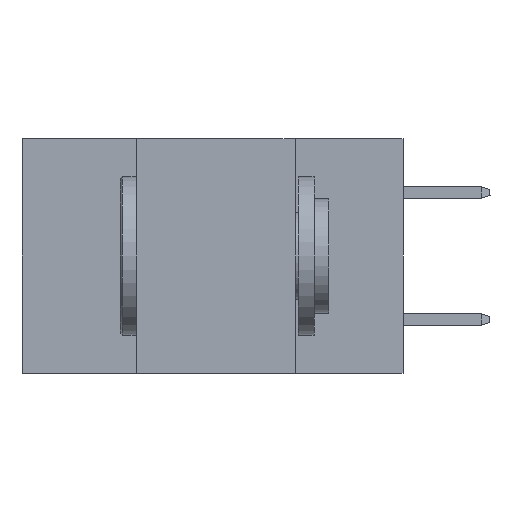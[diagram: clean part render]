
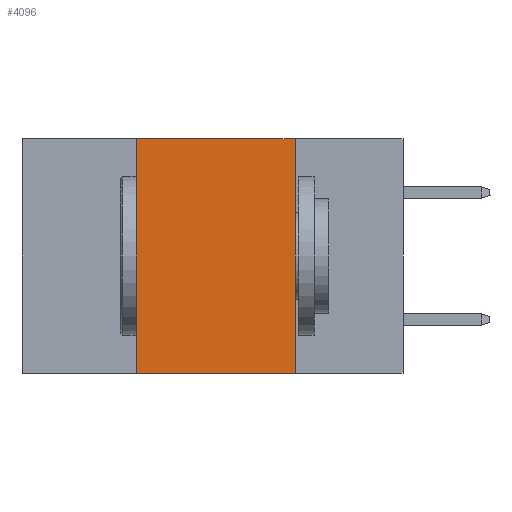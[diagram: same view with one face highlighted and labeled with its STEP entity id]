
A CAD part, left-side view. The second image highlights one B-rep face of the part: STEP entity #4096.
In plain terms, the highlighted planar face has unit normal (-1, 0, 0).
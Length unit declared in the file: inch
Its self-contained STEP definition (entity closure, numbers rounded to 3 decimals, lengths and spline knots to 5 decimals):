
#865 = ORIENTED_EDGE ( 'NONE', *, *, #6094, .F. ) ;
#1149 = EDGE_CURVE ( 'NONE', #20734, #7047, #16220, .T. ) ;
#1328 = DIRECTION ( 'NONE',  ( 1., 0., 0. ) ) ;
#2461 = EDGE_LOOP ( 'NONE', ( #10804, #13044, #865, #14451 ) ) ;
#4096 = ADVANCED_FACE ( 'NONE', ( #12224 ), #18848, .F. ) ;
#4247 = CARTESIAN_POINT ( 'NONE',  ( 0., 0.17, -0.37 ) ) ;
#5621 = VECTOR ( 'NONE', #19192, 39.37008 ) ;
#5815 = CARTESIAN_POINT ( 'NONE',  ( 0., 0.42, 0. ) ) ;
#6094 = EDGE_CURVE ( 'NONE', #20734, #10146, #17263, .T. ) ;
#6419 = CARTESIAN_POINT ( 'NONE',  ( 0., 0.6, -0.37 ) ) ;
#6500 = EDGE_CURVE ( 'NONE', #13744, #7047, #10813, .T. ) ;
#6738 = AXIS2_PLACEMENT_3D ( 'NONE', #15898, #1328, #8083 ) ;
#6905 = CARTESIAN_POINT ( 'NONE',  ( 0., 0.6, 0. ) ) ;
#7047 = VERTEX_POINT ( 'NONE', #4247 ) ;
#8083 = DIRECTION ( 'NONE',  ( 0., 0., -1. ) ) ;
#8757 = CARTESIAN_POINT ( 'NONE',  ( 0., 0.42, -0.37 ) ) ;
#9327 = DIRECTION ( 'NONE',  ( 0., 0., 1. ) ) ;
#9439 = VECTOR ( 'NONE', #9327, 39.37008 ) ;
#10146 = VERTEX_POINT ( 'NONE', #5815 ) ;
#10548 = CARTESIAN_POINT ( 'NONE',  ( 0., 0.17, 0. ) ) ;
#10804 = ORIENTED_EDGE ( 'NONE', *, *, #6500, .F. ) ;
#10813 = LINE ( 'NONE', #15384, #5621 ) ;
#12224 = FACE_OUTER_BOUND ( 'NONE', #2461, .T. ) ;
#13044 = ORIENTED_EDGE ( 'NONE', *, *, #17514, .F. ) ;
#13744 = VERTEX_POINT ( 'NONE', #10548 ) ;
#14451 = ORIENTED_EDGE ( 'NONE', *, *, #1149, .T. ) ;
#15201 = VECTOR ( 'NONE', #19949, 39.37008 ) ;
#15257 = VECTOR ( 'NONE', #18065, 39.37008 ) ;
#15384 = CARTESIAN_POINT ( 'NONE',  ( 0., 0.17, 0. ) ) ;
#15898 = CARTESIAN_POINT ( 'NONE',  ( 0., 0.6, 0. ) ) ;
#16220 = LINE ( 'NONE', #6419, #15257 ) ;
#17263 = LINE ( 'NONE', #17587, #9439 ) ;
#17514 = EDGE_CURVE ( 'NONE', #10146, #13744, #18112, .T. ) ;
#17587 = CARTESIAN_POINT ( 'NONE',  ( 0., 0.42, 0. ) ) ;
#18065 = DIRECTION ( 'NONE',  ( 0., -1., 0. ) ) ;
#18112 = LINE ( 'NONE', #6905, #15201 ) ;
#18848 = PLANE ( 'NONE',  #6738 ) ;
#19192 = DIRECTION ( 'NONE',  ( 0., 0., -1. ) ) ;
#19949 = DIRECTION ( 'NONE',  ( 0., -1., 0. ) ) ;
#20734 = VERTEX_POINT ( 'NONE', #8757 ) ;
